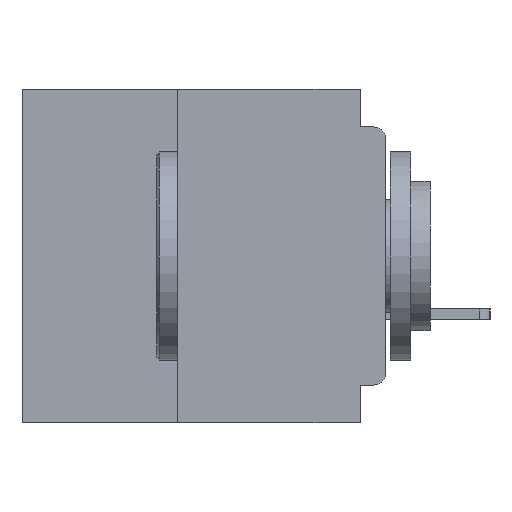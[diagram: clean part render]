
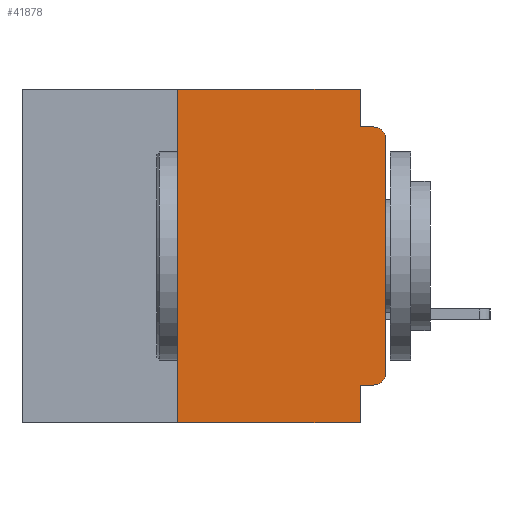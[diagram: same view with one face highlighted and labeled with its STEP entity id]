
A CAD part, left-side view. The second image highlights one B-rep face of the part: STEP entity #41878.
In plain terms, the highlighted planar face has unit normal (-1, 0, 0).
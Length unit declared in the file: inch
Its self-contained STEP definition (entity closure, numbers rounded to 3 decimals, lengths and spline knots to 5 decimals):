
#434 = VECTOR ( 'NONE', #40305, 39.37008 ) ;
#2189 = CARTESIAN_POINT ( 'NONE',  ( 0., 0.015, -0.34 ) ) ;
#2328 = CARTESIAN_POINT ( 'NONE',  ( 0., 0.25, -0.4 ) ) ;
#2396 = VERTEX_POINT ( 'NONE', #21483 ) ;
#2656 = CARTESIAN_POINT ( 'NONE',  ( 0., 0.031, 0. ) ) ;
#4050 = CARTESIAN_POINT ( 'NONE',  ( 0., 0.015, -0.06 ) ) ;
#4118 = CARTESIAN_POINT ( 'NONE',  ( 0., 0.031, -0.4 ) ) ;
#4187 = VERTEX_POINT ( 'NONE', #2656 ) ;
#5126 = LINE ( 'NONE', #27982, #22863 ) ;
#5333 = ORIENTED_EDGE ( 'NONE', *, *, #18935, .F. ) ;
#5568 = DIRECTION ( 'NONE',  ( 0., 0., -1. ) ) ;
#6186 = LINE ( 'NONE', #10911, #40599 ) ;
#7114 = EDGE_CURVE ( 'NONE', #4187, #18079, #9351, .T. ) ;
#7224 = DIRECTION ( 'NONE',  ( 0., 1., 0. ) ) ;
#7411 = DIRECTION ( 'NONE',  ( 0., 0., -1. ) ) ;
#7990 = DIRECTION ( 'NONE',  ( 0., 0., 1. ) ) ;
#8158 = CARTESIAN_POINT ( 'NONE',  ( 0., 0.437, -0.4 ) ) ;
#8701 = EDGE_CURVE ( 'NONE', #18079, #38972, #26424, .T. ) ;
#8712 = VECTOR ( 'NONE', #31508, 39.37008 ) ;
#9351 = LINE ( 'NONE', #20343, #434 ) ;
#10359 = EDGE_CURVE ( 'NONE', #21058, #4187, #6186, .T. ) ;
#10363 = EDGE_CURVE ( 'NONE', #26648, #2396, #5126, .T. ) ;
#10407 = CARTESIAN_POINT ( 'NONE',  ( 0., 0.015, -0.355 ) ) ;
#10911 = CARTESIAN_POINT ( 'NONE',  ( 0., 0.437, 0. ) ) ;
#11331 = DIRECTION ( 'NONE',  ( 0., 0., -1. ) ) ;
#12249 = AXIS2_PLACEMENT_3D ( 'NONE', #4050, #27396, #7411 ) ;
#12614 = VECTOR ( 'NONE', #11331, 39.37008 ) ;
#12717 = VERTEX_POINT ( 'NONE', #10407 ) ;
#14062 = VERTEX_POINT ( 'NONE', #16796 ) ;
#14161 = DIRECTION ( 'NONE',  ( 1., 0., 0. ) ) ;
#14573 = DIRECTION ( 'NONE',  ( 0., -1., 0. ) ) ;
#14744 = LINE ( 'NONE', #34708, #12614 ) ;
#14880 = CIRCLE ( 'NONE', #20003, 0.015 ) ;
#16251 = EDGE_CURVE ( 'NONE', #2396, #38972, #19251, .T. ) ;
#16796 = CARTESIAN_POINT ( 'NONE',  ( 0., 0.25, -0.4 ) ) ;
#17350 = CARTESIAN_POINT ( 'NONE',  ( 0., 0.031, -0.045 ) ) ;
#17607 = LINE ( 'NONE', #8158, #8712 ) ;
#18079 = VERTEX_POINT ( 'NONE', #17350 ) ;
#18935 = EDGE_CURVE ( 'NONE', #14062, #21058, #37397, .T. ) ;
#19251 = CIRCLE ( 'NONE', #12249, 0.015 ) ;
#20003 = AXIS2_PLACEMENT_3D ( 'NONE', #2189, #25546, #5568 ) ;
#20343 = CARTESIAN_POINT ( 'NONE',  ( 0., 0.031, 0. ) ) ;
#20493 = LINE ( 'NONE', #24003, #26221 ) ;
#21058 = VERTEX_POINT ( 'NONE', #21281 ) ;
#21281 = CARTESIAN_POINT ( 'NONE',  ( 0., 0.25, 0. ) ) ;
#21323 = EDGE_LOOP ( 'NONE', ( #43050, #41589, #32186, #23123, #36224, #5333, #39640, #33966, #27078, #23541 ) ) ;
#21483 = CARTESIAN_POINT ( 'NONE',  ( 0., 0., -0.06 ) ) ;
#22301 = DIRECTION ( 'NONE',  ( 0., 0., 1. ) ) ;
#22863 = VECTOR ( 'NONE', #7990, 39.37008 ) ;
#23123 = ORIENTED_EDGE ( 'NONE', *, *, #7114, .F. ) ;
#23541 = ORIENTED_EDGE ( 'NONE', *, *, #39317, .T. ) ;
#24003 = CARTESIAN_POINT ( 'NONE',  ( 0., 0., -0.355 ) ) ;
#24192 = FACE_OUTER_BOUND ( 'NONE', #21323, .T. ) ;
#25332 = EDGE_CURVE ( 'NONE', #12717, #34560, #20493, .T. ) ;
#25546 = DIRECTION ( 'NONE',  ( -1., 0., 0. ) ) ;
#26221 = VECTOR ( 'NONE', #7224, 39.37008 ) ;
#26424 = LINE ( 'NONE', #34693, #43057 ) ;
#26648 = VERTEX_POINT ( 'NONE', #34566 ) ;
#27078 = ORIENTED_EDGE ( 'NONE', *, *, #25332, .F. ) ;
#27271 = CARTESIAN_POINT ( 'NONE',  ( 0., 0.437, 0. ) ) ;
#27396 = DIRECTION ( 'NONE',  ( -1., 0., 0. ) ) ;
#27982 = CARTESIAN_POINT ( 'NONE',  ( 0., 0., 0. ) ) ;
#28502 = VECTOR ( 'NONE', #22301, 39.37008 ) ;
#30378 = CARTESIAN_POINT ( 'NONE',  ( 0., 0.015, -0.045 ) ) ;
#31309 = DIRECTION ( 'NONE',  ( 0., -1., 0. ) ) ;
#31508 = DIRECTION ( 'NONE',  ( 0., -1., 0. ) ) ;
#32186 = ORIENTED_EDGE ( 'NONE', *, *, #8701, .F. ) ;
#33966 = ORIENTED_EDGE ( 'NONE', *, *, #34558, .F. ) ;
#34154 = PLANE ( 'NONE',  #41567 ) ;
#34558 = EDGE_CURVE ( 'NONE', #34560, #41321, #14744, .T. ) ;
#34560 = VERTEX_POINT ( 'NONE', #37897 ) ;
#34566 = CARTESIAN_POINT ( 'NONE',  ( 0., 0., -0.34 ) ) ;
#34693 = CARTESIAN_POINT ( 'NONE',  ( 0., 0., -0.045 ) ) ;
#34708 = CARTESIAN_POINT ( 'NONE',  ( 0., 0.031, -0.4 ) ) ;
#36224 = ORIENTED_EDGE ( 'NONE', *, *, #10359, .F. ) ;
#37397 = LINE ( 'NONE', #2328, #28502 ) ;
#37465 = EDGE_CURVE ( 'NONE', #14062, #41321, #17607, .T. ) ;
#37502 = DIRECTION ( 'NONE',  ( 0., 0., -1. ) ) ;
#37897 = CARTESIAN_POINT ( 'NONE',  ( 0., 0.031, -0.355 ) ) ;
#38972 = VERTEX_POINT ( 'NONE', #30378 ) ;
#39317 = EDGE_CURVE ( 'NONE', #12717, #26648, #14880, .T. ) ;
#39640 = ORIENTED_EDGE ( 'NONE', *, *, #37465, .T. ) ;
#40305 = DIRECTION ( 'NONE',  ( 0., 0., -1. ) ) ;
#40599 = VECTOR ( 'NONE', #14573, 39.37008 ) ;
#41321 = VERTEX_POINT ( 'NONE', #4118 ) ;
#41567 = AXIS2_PLACEMENT_3D ( 'NONE', #27271, #14161, #37502 ) ;
#41589 = ORIENTED_EDGE ( 'NONE', *, *, #16251, .T. ) ;
#41878 = ADVANCED_FACE ( 'NONE', ( #24192 ), #34154, .F. ) ;
#43050 = ORIENTED_EDGE ( 'NONE', *, *, #10363, .T. ) ;
#43057 = VECTOR ( 'NONE', #31309, 39.37008 ) ;
